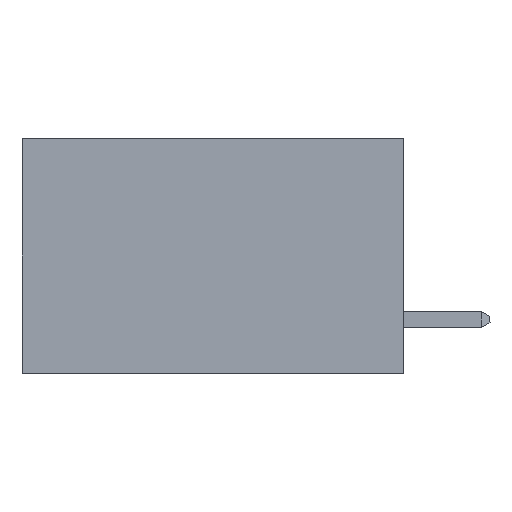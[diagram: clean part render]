
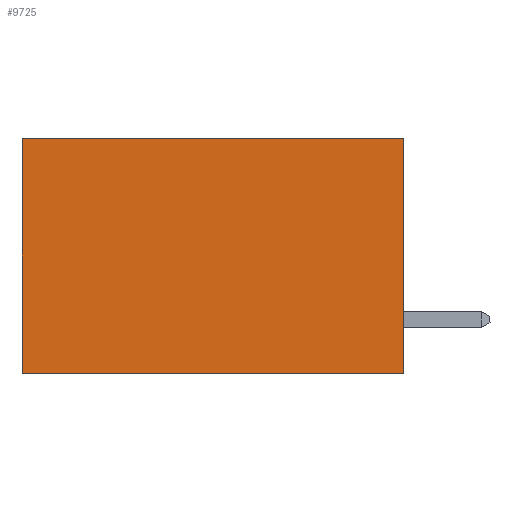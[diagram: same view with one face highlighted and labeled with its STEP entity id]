
A CAD part, left-side view. The second image highlights one B-rep face of the part: STEP entity #9725.
In plain terms, the highlighted planar face has unit normal (-1, 0, 0).
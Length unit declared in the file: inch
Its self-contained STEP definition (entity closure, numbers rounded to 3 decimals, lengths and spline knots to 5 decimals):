
#1117 = EDGE_LOOP ( 'NONE', ( #7150, #7346, #7533, #4393 ) ) ;
#2230 = EDGE_CURVE ( 'NONE', #16174, #5270, #2883, .T. ) ;
#2281 = PLANE ( 'NONE',  #16677 ) ;
#2407 = DIRECTION ( 'NONE',  ( 0., 1., 0. ) ) ;
#2883 = LINE ( 'NONE', #8805, #9592 ) ;
#2952 = VERTEX_POINT ( 'NONE', #4088 ) ;
#3646 = DIRECTION ( 'NONE',  ( 1., 0., 0. ) ) ;
#3665 = CARTESIAN_POINT ( 'NONE',  ( 0.2875, 0.6, 0. ) ) ;
#3701 = CARTESIAN_POINT ( 'NONE',  ( 0.2875, 0., 0. ) ) ;
#3910 = VECTOR ( 'NONE', #14043, 39.37008 ) ;
#3969 = CARTESIAN_POINT ( 'NONE',  ( 0.2875, 0.6, -0.37 ) ) ;
#4088 = CARTESIAN_POINT ( 'NONE',  ( 0.2875, 0., 0. ) ) ;
#4328 = LINE ( 'NONE', #12778, #3910 ) ;
#4393 = ORIENTED_EDGE ( 'NONE', *, *, #4473, .T. ) ;
#4473 = EDGE_CURVE ( 'NONE', #2952, #7209, #9180, .T. ) ;
#4663 = VECTOR ( 'NONE', #10270, 39.37008 ) ;
#5270 = VERTEX_POINT ( 'NONE', #3969 ) ;
#7150 = ORIENTED_EDGE ( 'NONE', *, *, #14859, .T. ) ;
#7209 = VERTEX_POINT ( 'NONE', #3665 ) ;
#7346 = ORIENTED_EDGE ( 'NONE', *, *, #2230, .F. ) ;
#7533 = ORIENTED_EDGE ( 'NONE', *, *, #7753, .F. ) ;
#7753 = EDGE_CURVE ( 'NONE', #2952, #16174, #12157, .T. ) ;
#8332 = DIRECTION ( 'NONE',  ( 0., 1., 0. ) ) ;
#8575 = VECTOR ( 'NONE', #2407, 39.37008 ) ;
#8805 = CARTESIAN_POINT ( 'NONE',  ( 0.2875, 0., -0.37 ) ) ;
#8941 = CARTESIAN_POINT ( 'NONE',  ( 0.2875, 0., 0. ) ) ;
#9180 = LINE ( 'NONE', #3701, #8575 ) ;
#9592 = VECTOR ( 'NONE', #8332, 39.37008 ) ;
#9725 = ADVANCED_FACE ( 'NONE', ( #16738 ), #2281, .F. ) ;
#10270 = DIRECTION ( 'NONE',  ( 0., 0., -1. ) ) ;
#11634 = CARTESIAN_POINT ( 'NONE',  ( 0.2875, 0., 0. ) ) ;
#12157 = LINE ( 'NONE', #8941, #4663 ) ;
#12778 = CARTESIAN_POINT ( 'NONE',  ( 0.2875, 0.6, 0. ) ) ;
#12911 = DIRECTION ( 'NONE',  ( 0., 0., -1. ) ) ;
#13933 = CARTESIAN_POINT ( 'NONE',  ( 0.2875, 0., -0.37 ) ) ;
#14043 = DIRECTION ( 'NONE',  ( 0., 0., -1. ) ) ;
#14859 = EDGE_CURVE ( 'NONE', #7209, #5270, #4328, .T. ) ;
#16174 = VERTEX_POINT ( 'NONE', #13933 ) ;
#16677 = AXIS2_PLACEMENT_3D ( 'NONE', #11634, #3646, #12911 ) ;
#16738 = FACE_OUTER_BOUND ( 'NONE', #1117, .T. ) ;
